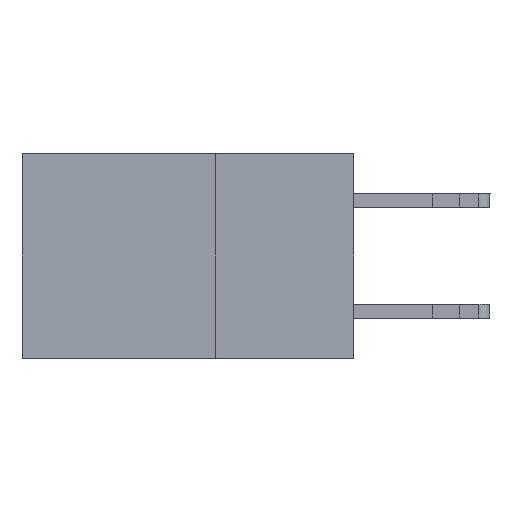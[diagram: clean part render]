
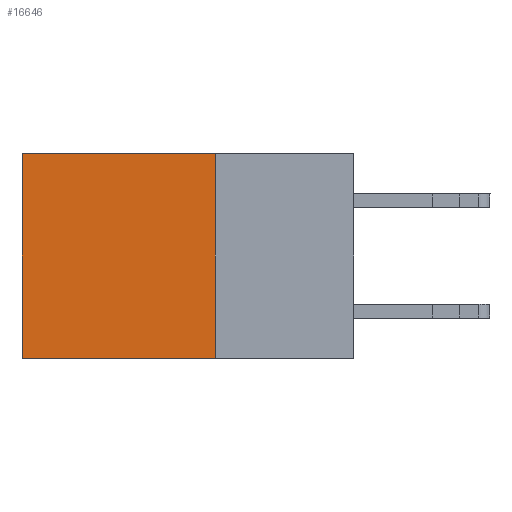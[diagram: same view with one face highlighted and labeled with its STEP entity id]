
A CAD part, left-side view. The second image highlights one B-rep face of the part: STEP entity #16646.
In plain terms, the highlighted planar face has unit normal (-1, 0, 0).
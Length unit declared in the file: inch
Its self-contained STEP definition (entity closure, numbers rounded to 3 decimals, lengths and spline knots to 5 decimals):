
#427 = PLANE ( 'NONE',  #18574 ) ;
#557 = VECTOR ( 'NONE', #5019, 39.37008 ) ;
#1631 = CARTESIAN_POINT ( 'NONE',  ( 0.2875, 0.6, 0. ) ) ;
#3680 = CARTESIAN_POINT ( 'NONE',  ( 0.2875, 0.25, 0. ) ) ;
#3985 = CARTESIAN_POINT ( 'NONE',  ( 0.2875, 0.25, -0.37 ) ) ;
#4073 = ORIENTED_EDGE ( 'NONE', *, *, #25319, .T. ) ;
#5019 = DIRECTION ( 'NONE',  ( 0., 1., 0. ) ) ;
#5192 = ORIENTED_EDGE ( 'NONE', *, *, #6253, .F. ) ;
#5675 = DIRECTION ( 'NONE',  ( 0., 1., 0. ) ) ;
#5764 = EDGE_CURVE ( 'NONE', #23841, #21172, #16413, .T. ) ;
#6253 = EDGE_CURVE ( 'NONE', #14346, #23361, #15155, .T. ) ;
#6374 = CARTESIAN_POINT ( 'NONE',  ( 0.2875, 0.25, 0. ) ) ;
#7660 = CARTESIAN_POINT ( 'NONE',  ( 0.2875, 0.6, 0. ) ) ;
#8082 = EDGE_CURVE ( 'NONE', #23361, #21172, #21580, .T. ) ;
#8363 = DIRECTION ( 'NONE',  ( 1., 0., 0. ) ) ;
#9753 = ORIENTED_EDGE ( 'NONE', *, *, #8082, .F. ) ;
#9906 = VECTOR ( 'NONE', #25370, 39.37008 ) ;
#11777 = VECTOR ( 'NONE', #21478, 39.37008 ) ;
#14023 = VECTOR ( 'NONE', #5675, 39.37008 ) ;
#14346 = VERTEX_POINT ( 'NONE', #25354 ) ;
#14653 = LINE ( 'NONE', #3680, #14023 ) ;
#15155 = LINE ( 'NONE', #17366, #9906 ) ;
#15788 = FACE_OUTER_BOUND ( 'NONE', #16779, .T. ) ;
#16413 = LINE ( 'NONE', #7660, #11777 ) ;
#16646 = ADVANCED_FACE ( 'NONE', ( #15788 ), #427, .F. ) ;
#16779 = EDGE_LOOP ( 'NONE', ( #21916, #9753, #5192, #4073 ) ) ;
#17366 = CARTESIAN_POINT ( 'NONE',  ( 0.2875, 0.25, 0. ) ) ;
#18574 = AXIS2_PLACEMENT_3D ( 'NONE', #6374, #8363, #22195 ) ;
#19111 = CARTESIAN_POINT ( 'NONE',  ( 0.2875, 0.6, -0.37 ) ) ;
#21172 = VERTEX_POINT ( 'NONE', #19111 ) ;
#21478 = DIRECTION ( 'NONE',  ( 0., 0., -1. ) ) ;
#21580 = LINE ( 'NONE', #24749, #557 ) ;
#21916 = ORIENTED_EDGE ( 'NONE', *, *, #5764, .T. ) ;
#22195 = DIRECTION ( 'NONE',  ( 0., 0., -1. ) ) ;
#23361 = VERTEX_POINT ( 'NONE', #3985 ) ;
#23841 = VERTEX_POINT ( 'NONE', #1631 ) ;
#24749 = CARTESIAN_POINT ( 'NONE',  ( 0.2875, 0.25, -0.37 ) ) ;
#25319 = EDGE_CURVE ( 'NONE', #14346, #23841, #14653, .T. ) ;
#25354 = CARTESIAN_POINT ( 'NONE',  ( 0.2875, 0.25, 0. ) ) ;
#25370 = DIRECTION ( 'NONE',  ( 0., 0., -1. ) ) ;
